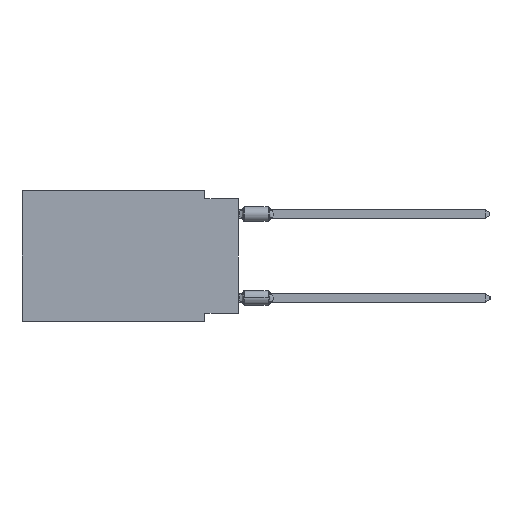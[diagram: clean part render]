
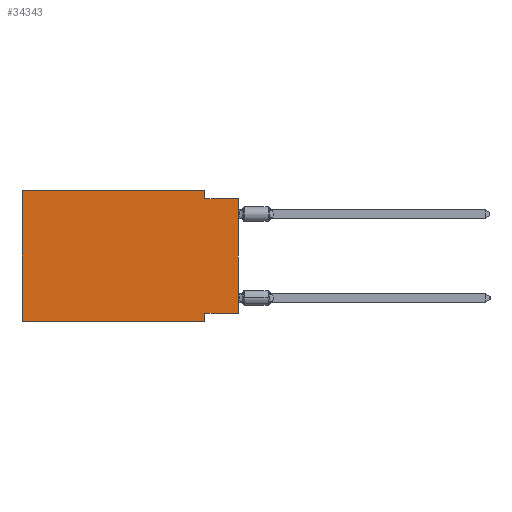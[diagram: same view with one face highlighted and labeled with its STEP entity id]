
A CAD part, left-side view. The second image highlights one B-rep face of the part: STEP entity #34343.
In plain terms, the highlighted planar face has unit normal (-1, 0, 0).
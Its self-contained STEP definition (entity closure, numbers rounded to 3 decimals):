
#579 = PLANE ( 'NONE',  #15582 ) ;
#1213 = CARTESIAN_POINT ( 'NONE',  ( 0., 2.54, -9.906 ) ) ;
#1397 = ORIENTED_EDGE ( 'NONE', *, *, #37665, .T. ) ;
#1474 = VECTOR ( 'NONE', #39852, 1000. ) ;
#1495 = VERTEX_POINT ( 'NONE', #32445 ) ;
#1985 = EDGE_CURVE ( 'NONE', #29860, #8379, #25091, .T. ) ;
#2704 = LINE ( 'NONE', #16218, #38924 ) ;
#2807 = DIRECTION ( 'NONE',  ( 0., -1., 0. ) ) ;
#3203 = EDGE_CURVE ( 'NONE', #10493, #38878, #5610, .T. ) ;
#3649 = VECTOR ( 'NONE', #22364, 1000. ) ;
#4782 = CARTESIAN_POINT ( 'NONE',  ( 0., 2.54, -9.271 ) ) ;
#5251 = CARTESIAN_POINT ( 'NONE',  ( 0., 16.383, 0. ) ) ;
#5340 = LINE ( 'NONE', #28360, #3649 ) ;
#5610 = LINE ( 'NONE', #29070, #41215 ) ;
#7458 = CARTESIAN_POINT ( 'NONE',  ( 0., 16.383, 0. ) ) ;
#7958 = VERTEX_POINT ( 'NONE', #1213 ) ;
#8154 = CARTESIAN_POINT ( 'NONE',  ( 0., 16.383, -9.906 ) ) ;
#8379 = VERTEX_POINT ( 'NONE', #10912 ) ;
#8919 = ORIENTED_EDGE ( 'NONE', *, *, #38703, .F. ) ;
#9974 = CARTESIAN_POINT ( 'NONE',  ( 0., 2.54, 0. ) ) ;
#10493 = VERTEX_POINT ( 'NONE', #8154 ) ;
#10851 = LINE ( 'NONE', #17697, #14186 ) ;
#10912 = CARTESIAN_POINT ( 'NONE',  ( 0., 0., -0.635 ) ) ;
#11262 = VERTEX_POINT ( 'NONE', #9974 ) ;
#11885 = DIRECTION ( 'NONE',  ( 0., -1., 0. ) ) ;
#12406 = CARTESIAN_POINT ( 'NONE',  ( 0., 16.383, 0. ) ) ;
#13047 = LINE ( 'NONE', #26321, #1474 ) ;
#13521 = ORIENTED_EDGE ( 'NONE', *, *, #24962, .F. ) ;
#13901 = EDGE_CURVE ( 'NONE', #11262, #29860, #2704, .T. ) ;
#14186 = VECTOR ( 'NONE', #21472, 1000. ) ;
#15582 = AXIS2_PLACEMENT_3D ( 'NONE', #7458, #33372, #20952 ) ;
#16218 = CARTESIAN_POINT ( 'NONE',  ( 0., 2.54, 0. ) ) ;
#17697 = CARTESIAN_POINT ( 'NONE',  ( 0., 0., -9.271 ) ) ;
#20515 = ORIENTED_EDGE ( 'NONE', *, *, #1985, .F. ) ;
#20952 = DIRECTION ( 'NONE',  ( 0., 0., -1. ) ) ;
#21472 = DIRECTION ( 'NONE',  ( 0., 1., 0. ) ) ;
#22272 = CARTESIAN_POINT ( 'NONE',  ( 0., 2.54, -0.635 ) ) ;
#22364 = DIRECTION ( 'NONE',  ( 0., 0., -1. ) ) ;
#22624 = DIRECTION ( 'NONE',  ( 0., 0., 1. ) ) ;
#23193 = EDGE_CURVE ( 'NONE', #38878, #11262, #38895, .T. ) ;
#23493 = VECTOR ( 'NONE', #2807, 1000. ) ;
#24962 = EDGE_CURVE ( 'NONE', #1495, #41142, #10851, .T. ) ;
#25091 = LINE ( 'NONE', #32986, #27682 ) ;
#25846 = CARTESIAN_POINT ( 'NONE',  ( 0., 16.383, -9.906 ) ) ;
#25908 = ORIENTED_EDGE ( 'NONE', *, *, #39228, .T. ) ;
#26321 = CARTESIAN_POINT ( 'NONE',  ( 0., 0., 0. ) ) ;
#27369 = FACE_OUTER_BOUND ( 'NONE', #34245, .T. ) ;
#27682 = VECTOR ( 'NONE', #35299, 1000. ) ;
#28360 = CARTESIAN_POINT ( 'NONE',  ( 0., 2.54, -9.906 ) ) ;
#29070 = CARTESIAN_POINT ( 'NONE',  ( 0., 16.383, 0. ) ) ;
#29860 = VERTEX_POINT ( 'NONE', #22272 ) ;
#29946 = VECTOR ( 'NONE', #11885, 1000. ) ;
#30291 = ORIENTED_EDGE ( 'NONE', *, *, #23193, .F. ) ;
#31305 = ORIENTED_EDGE ( 'NONE', *, *, #3203, .F. ) ;
#32445 = CARTESIAN_POINT ( 'NONE',  ( 0., 0., -9.271 ) ) ;
#32986 = CARTESIAN_POINT ( 'NONE',  ( 0., 0., -0.635 ) ) ;
#33149 = LINE ( 'NONE', #25846, #23493 ) ;
#33372 = DIRECTION ( 'NONE',  ( 1., 0., 0. ) ) ;
#34245 = EDGE_LOOP ( 'NONE', ( #1397, #20515, #43690, #30291, #31305, #25908, #8919, #13521 ) ) ;
#34343 = ADVANCED_FACE ( 'NONE', ( #27369 ), #579, .F. ) ;
#35299 = DIRECTION ( 'NONE',  ( 0., -1., 0. ) ) ;
#37665 = EDGE_CURVE ( 'NONE', #1495, #8379, #13047, .T. ) ;
#38703 = EDGE_CURVE ( 'NONE', #41142, #7958, #5340, .T. ) ;
#38878 = VERTEX_POINT ( 'NONE', #12406 ) ;
#38895 = LINE ( 'NONE', #5251, #29946 ) ;
#38924 = VECTOR ( 'NONE', #43234, 1000. ) ;
#39228 = EDGE_CURVE ( 'NONE', #10493, #7958, #33149, .T. ) ;
#39852 = DIRECTION ( 'NONE',  ( 0., 0., 1. ) ) ;
#41142 = VERTEX_POINT ( 'NONE', #4782 ) ;
#41215 = VECTOR ( 'NONE', #22624, 1000. ) ;
#43234 = DIRECTION ( 'NONE',  ( 0., 0., -1. ) ) ;
#43690 = ORIENTED_EDGE ( 'NONE', *, *, #13901, .F. ) ;
